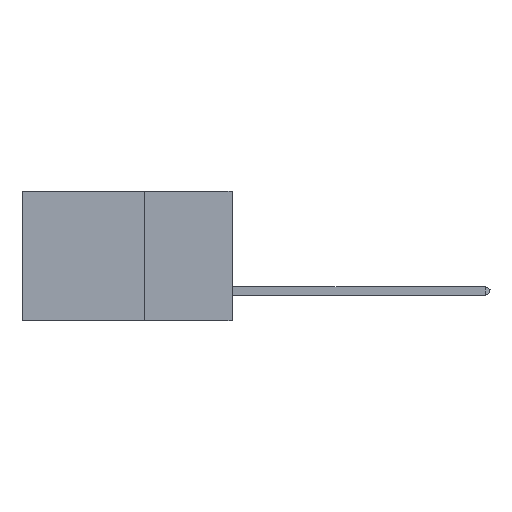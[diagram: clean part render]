
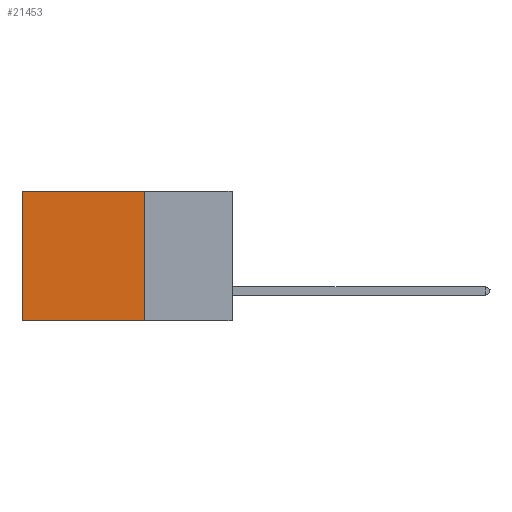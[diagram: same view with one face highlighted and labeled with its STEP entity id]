
A CAD part, left-side view. The second image highlights one B-rep face of the part: STEP entity #21453.
In plain terms, the highlighted planar face has unit normal (-1, 0, 0).
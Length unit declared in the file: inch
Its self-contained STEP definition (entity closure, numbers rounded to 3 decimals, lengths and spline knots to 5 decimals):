
#2503 = CARTESIAN_POINT ( 'NONE',  ( 0.2875, 0.6, 0. ) ) ;
#2673 = AXIS2_PLACEMENT_3D ( 'NONE', #23801, #6642, #30512 ) ;
#4994 = CARTESIAN_POINT ( 'NONE',  ( 0.2875, 0.25, -0.37 ) ) ;
#6523 = FACE_OUTER_BOUND ( 'NONE', #6707, .T. ) ;
#6642 = DIRECTION ( 'NONE',  ( 1., 0., 0. ) ) ;
#6707 = EDGE_LOOP ( 'NONE', ( #26690, #17333, #37207, #22428 ) ) ;
#8376 = CARTESIAN_POINT ( 'NONE',  ( 0.2875, 0.6, -0.37 ) ) ;
#9378 = EDGE_CURVE ( 'NONE', #35622, #39009, #32877, .T. ) ;
#10373 = EDGE_CURVE ( 'NONE', #40024, #35622, #10462, .T. ) ;
#10462 = LINE ( 'NONE', #30130, #18436 ) ;
#12610 = CARTESIAN_POINT ( 'NONE',  ( 0.2875, 0.25, 0. ) ) ;
#16563 = VERTEX_POINT ( 'NONE', #4994 ) ;
#17333 = ORIENTED_EDGE ( 'NONE', *, *, #40347, .F. ) ;
#17700 = EDGE_CURVE ( 'NONE', #40024, #16563, #39298, .T. ) ;
#18436 = VECTOR ( 'NONE', #35109, 39.37008 ) ;
#21453 = ADVANCED_FACE ( 'NONE', ( #6523 ), #32816, .F. ) ;
#22428 = ORIENTED_EDGE ( 'NONE', *, *, #10373, .T. ) ;
#23801 = CARTESIAN_POINT ( 'NONE',  ( 0.2875, 0.25, 0. ) ) ;
#23984 = DIRECTION ( 'NONE',  ( 0., 1., 0. ) ) ;
#24120 = CARTESIAN_POINT ( 'NONE',  ( 0.2875, 0.25, -0.37 ) ) ;
#24278 = VECTOR ( 'NONE', #23984, 39.37008 ) ;
#24807 = CARTESIAN_POINT ( 'NONE',  ( 0.2875, 0.6, 0. ) ) ;
#26690 = ORIENTED_EDGE ( 'NONE', *, *, #9378, .T. ) ;
#30130 = CARTESIAN_POINT ( 'NONE',  ( 0.2875, 0.25, 0. ) ) ;
#30307 = VECTOR ( 'NONE', #40330, 39.37008 ) ;
#30512 = DIRECTION ( 'NONE',  ( 0., 0., -1. ) ) ;
#30533 = CARTESIAN_POINT ( 'NONE',  ( 0.2875, 0.25, 0. ) ) ;
#32816 = PLANE ( 'NONE',  #2673 ) ;
#32877 = LINE ( 'NONE', #2503, #37067 ) ;
#35109 = DIRECTION ( 'NONE',  ( 0., 1., 0. ) ) ;
#35622 = VERTEX_POINT ( 'NONE', #24807 ) ;
#36731 = DIRECTION ( 'NONE',  ( 0., 0., -1. ) ) ;
#37067 = VECTOR ( 'NONE', #36731, 39.37008 ) ;
#37207 = ORIENTED_EDGE ( 'NONE', *, *, #17700, .F. ) ;
#39009 = VERTEX_POINT ( 'NONE', #8376 ) ;
#39298 = LINE ( 'NONE', #30533, #30307 ) ;
#40024 = VERTEX_POINT ( 'NONE', #12610 ) ;
#40330 = DIRECTION ( 'NONE',  ( 0., 0., -1. ) ) ;
#40347 = EDGE_CURVE ( 'NONE', #16563, #39009, #43492, .T. ) ;
#43492 = LINE ( 'NONE', #24120, #24278 ) ;
